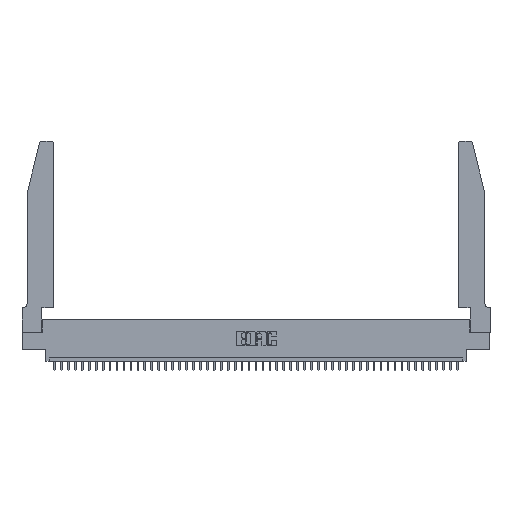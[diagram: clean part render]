
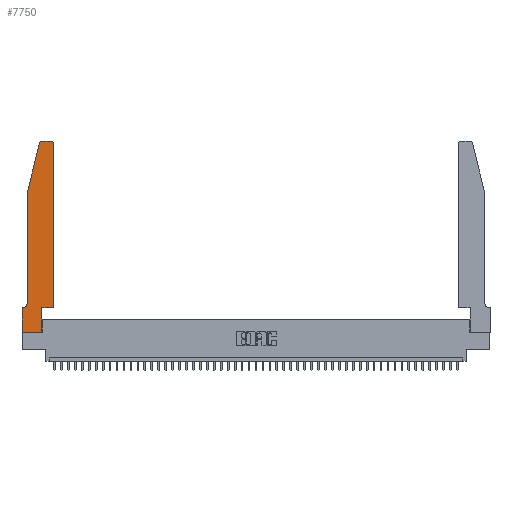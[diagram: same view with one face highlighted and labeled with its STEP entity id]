
A CAD part, top view. The second image highlights one B-rep face of the part: STEP entity #7750.
In plain terms, the highlighted planar face has unit normal (0, 0, 1).
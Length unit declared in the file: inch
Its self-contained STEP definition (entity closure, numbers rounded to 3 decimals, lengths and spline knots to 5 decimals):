
#17 = CARTESIAN_POINT ( 'NONE',  ( 0., 0., 0.37 ) ) ;
#135 = ORIENTED_EDGE ( 'NONE', *, *, #8508, .T. ) ;
#2735 = CARTESIAN_POINT ( 'NONE',  ( 0.0055, 0.35, 0.37 ) ) ;
#2770 = AXIS2_PLACEMENT_3D ( 'NONE', #27698, #31483, #27551 ) ;
#3969 = VERTEX_POINT ( 'NONE', #33456 ) ;
#4226 = ORIENTED_EDGE ( 'NONE', *, *, #33858, .T. ) ;
#4439 = EDGE_CURVE ( 'NONE', #24036, #46952, #17188, .T. ) ;
#5043 = CIRCLE ( 'NONE', #9810, 0.03 ) ;
#5192 = EDGE_CURVE ( 'NONE', #28645, #24795, #10957, .T. ) ;
#5860 = ORIENTED_EDGE ( 'NONE', *, *, #44178, .T. ) ;
#5964 = DIRECTION ( 'NONE',  ( 0., 0., 1. ) ) ;
#6250 = VERTEX_POINT ( 'NONE', #9262 ) ;
#6366 = CARTESIAN_POINT ( 'NONE',  ( 0.284, 2.72, 0.37 ) ) ;
#6711 = LINE ( 'NONE', #33224, #37912 ) ;
#7442 = VERTEX_POINT ( 'NONE', #21757 ) ;
#7750 = ADVANCED_FACE ( 'NONE', ( #20356 ), #25363, .T. ) ;
#8162 = VECTOR ( 'NONE', #18546, 39.37008 ) ;
#8508 = EDGE_CURVE ( 'NONE', #45870, #7442, #16303, .T. ) ;
#8727 = LINE ( 'NONE', #27396, #41647 ) ;
#8758 = CARTESIAN_POINT ( 'NONE',  ( 0.2605, 2.75, 0.37 ) ) ;
#9262 = CARTESIAN_POINT ( 'NONE',  ( 0., 0., 0.37 ) ) ;
#9512 = ORIENTED_EDGE ( 'NONE', *, *, #40230, .T. ) ;
#9810 = AXIS2_PLACEMENT_3D ( 'NONE', #34539, #5964, #30875 ) ;
#10508 = CARTESIAN_POINT ( 'NONE',  ( 0.0755, 2., 0.37 ) ) ;
#10957 = LINE ( 'NONE', #26623, #35318 ) ;
#10980 = VECTOR ( 'NONE', #37751, 39.37008 ) ;
#11030 = EDGE_CURVE ( 'NONE', #6250, #3969, #13909, .T. ) ;
#11579 = CARTESIAN_POINT ( 'NONE',  ( 0., 0., 0.37 ) ) ;
#11676 = DIRECTION ( 'NONE',  ( 0., 1., 0. ) ) ;
#13052 = CARTESIAN_POINT ( 'NONE',  ( 0.284, 2.75, 0.37 ) ) ;
#13657 = DIRECTION ( 'NONE',  ( 1., 0., 0. ) ) ;
#13900 = CIRCLE ( 'NONE', #2770, 0.07 ) ;
#13909 = LINE ( 'NONE', #11579, #8162 ) ;
#15999 = CARTESIAN_POINT ( 'NONE',  ( 0.0755, 0.35, 0.37 ) ) ;
#16158 = CARTESIAN_POINT ( 'NONE',  ( 0.0755, 2., 0.37 ) ) ;
#16303 = LINE ( 'NONE', #15999, #17432 ) ;
#16624 = EDGE_LOOP ( 'NONE', ( #32583, #4226, #20285, #9512, #33945, #135, #40120, #28030, #45025, #18224, #21956, #5860 ) ) ;
#17188 = LINE ( 'NONE', #24947, #25765 ) ;
#17391 = DIRECTION ( 'NONE',  ( 1., 0., 0. ) ) ;
#17432 = VECTOR ( 'NONE', #22688, 39.37008 ) ;
#18224 = ORIENTED_EDGE ( 'NONE', *, *, #5192, .T. ) ;
#18530 = CARTESIAN_POINT ( 'NONE',  ( 0.0755, 0.42, 0.37 ) ) ;
#18546 = DIRECTION ( 'NONE',  ( 1., 0., 0. ) ) ;
#19345 = VERTEX_POINT ( 'NONE', #13052 ) ;
#20285 = ORIENTED_EDGE ( 'NONE', *, *, #4439, .T. ) ;
#20356 = FACE_OUTER_BOUND ( 'NONE', #16624, .T. ) ;
#21227 = CARTESIAN_POINT ( 'NONE',  ( 0., 0.35, 0.37 ) ) ;
#21757 = CARTESIAN_POINT ( 'NONE',  ( 0., 0.35, 0.37 ) ) ;
#21956 = ORIENTED_EDGE ( 'NONE', *, *, #35405, .T. ) ;
#21974 = CIRCLE ( 'NONE', #38754, 0.03 ) ;
#22648 = CARTESIAN_POINT ( 'NONE',  ( 0.4205, 2.75, 0.37 ) ) ;
#22688 = DIRECTION ( 'NONE',  ( -1., 0., 0. ) ) ;
#24036 = VERTEX_POINT ( 'NONE', #25235 ) ;
#24554 = LINE ( 'NONE', #17, #35325 ) ;
#24795 = VERTEX_POINT ( 'NONE', #44035 ) ;
#24800 = EDGE_CURVE ( 'NONE', #3969, #28645, #6711, .T. ) ;
#24947 = CARTESIAN_POINT ( 'NONE',  ( 0.0755, 2., 0.37 ) ) ;
#25235 = CARTESIAN_POINT ( 'NONE',  ( 0.25487, 2.72718, 0.37 ) ) ;
#25363 = PLANE ( 'NONE',  #38977 ) ;
#25730 = CARTESIAN_POINT ( 'NONE',  ( 0.2865, 0.35, 0.37 ) ) ;
#25765 = VECTOR ( 'NONE', #28261, 39.37008 ) ;
#26623 = CARTESIAN_POINT ( 'NONE',  ( 0.4505, 0.35, 0.37 ) ) ;
#27396 = CARTESIAN_POINT ( 'NONE',  ( 0.4505, 0.35, 0.37 ) ) ;
#27551 = DIRECTION ( 'NONE',  ( -1., 0., 0. ) ) ;
#27698 = CARTESIAN_POINT ( 'NONE',  ( 0.0055, 0.42, 0.37 ) ) ;
#28030 = ORIENTED_EDGE ( 'NONE', *, *, #11030, .T. ) ;
#28261 = DIRECTION ( 'NONE',  ( -0.239, -0.971, 0. ) ) ;
#28303 = EDGE_CURVE ( 'NONE', #29729, #19345, #30255, .T. ) ;
#28645 = VERTEX_POINT ( 'NONE', #25730 ) ;
#29729 = VERTEX_POINT ( 'NONE', #22648 ) ;
#30255 = LINE ( 'NONE', #8758, #10980 ) ;
#30745 = DIRECTION ( 'NONE',  ( 0., -1., 0. ) ) ;
#30875 = DIRECTION ( 'NONE',  ( 1., 0., 0. ) ) ;
#31483 = DIRECTION ( 'NONE',  ( 0., 0., -1. ) ) ;
#32583 = ORIENTED_EDGE ( 'NONE', *, *, #28303, .T. ) ;
#32823 = DIRECTION ( 'NONE',  ( 0., -1., 0. ) ) ;
#33224 = CARTESIAN_POINT ( 'NONE',  ( 0.2865, 0.35, 0.37 ) ) ;
#33456 = CARTESIAN_POINT ( 'NONE',  ( 0.2865, 0., 0.37 ) ) ;
#33858 = EDGE_CURVE ( 'NONE', #19345, #24036, #21974, .T. ) ;
#33945 = ORIENTED_EDGE ( 'NONE', *, *, #40779, .T. ) ;
#34539 = CARTESIAN_POINT ( 'NONE',  ( 0.4205, 2.72, 0.37 ) ) ;
#34964 = VECTOR ( 'NONE', #30745, 39.37008 ) ;
#35083 = CARTESIAN_POINT ( 'NONE',  ( 0.4505, 2.72, 0.37 ) ) ;
#35318 = VECTOR ( 'NONE', #40584, 39.37008 ) ;
#35325 = VECTOR ( 'NONE', #32823, 39.37008 ) ;
#35405 = EDGE_CURVE ( 'NONE', #24795, #45886, #8727, .T. ) ;
#35655 = DIRECTION ( 'NONE',  ( 0., 0., 1. ) ) ;
#35715 = DIRECTION ( 'NONE',  ( 0., 0., 1. ) ) ;
#36652 = VERTEX_POINT ( 'NONE', #18530 ) ;
#36665 = LINE ( 'NONE', #16158, #34964 ) ;
#37751 = DIRECTION ( 'NONE',  ( -1., 0., 0. ) ) ;
#37912 = VECTOR ( 'NONE', #11676, 39.37008 ) ;
#37993 = DIRECTION ( 'NONE',  ( 0., 1., 0. ) ) ;
#38754 = AXIS2_PLACEMENT_3D ( 'NONE', #6366, #35715, #13657 ) ;
#38977 = AXIS2_PLACEMENT_3D ( 'NONE', #21227, #35655, #17391 ) ;
#40120 = ORIENTED_EDGE ( 'NONE', *, *, #41777, .T. ) ;
#40230 = EDGE_CURVE ( 'NONE', #46952, #36652, #36665, .T. ) ;
#40584 = DIRECTION ( 'NONE',  ( 1., 0., 0. ) ) ;
#40779 = EDGE_CURVE ( 'NONE', #36652, #45870, #13900, .T. ) ;
#41647 = VECTOR ( 'NONE', #37993, 39.37008 ) ;
#41777 = EDGE_CURVE ( 'NONE', #7442, #6250, #24554, .T. ) ;
#44035 = CARTESIAN_POINT ( 'NONE',  ( 0.4505, 0.35, 0.37 ) ) ;
#44178 = EDGE_CURVE ( 'NONE', #45886, #29729, #5043, .T. ) ;
#45025 = ORIENTED_EDGE ( 'NONE', *, *, #24800, .T. ) ;
#45870 = VERTEX_POINT ( 'NONE', #2735 ) ;
#45886 = VERTEX_POINT ( 'NONE', #35083 ) ;
#46952 = VERTEX_POINT ( 'NONE', #10508 ) ;
